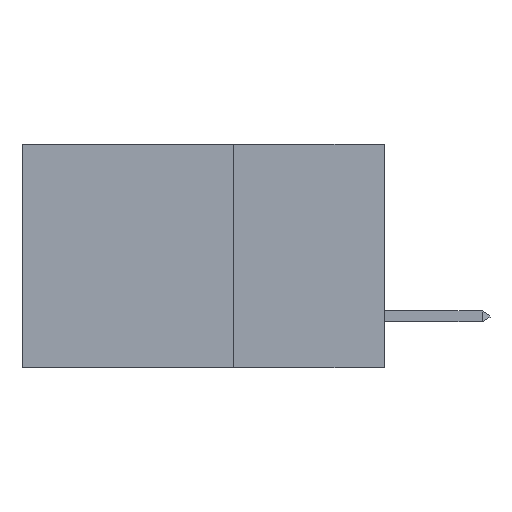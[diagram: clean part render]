
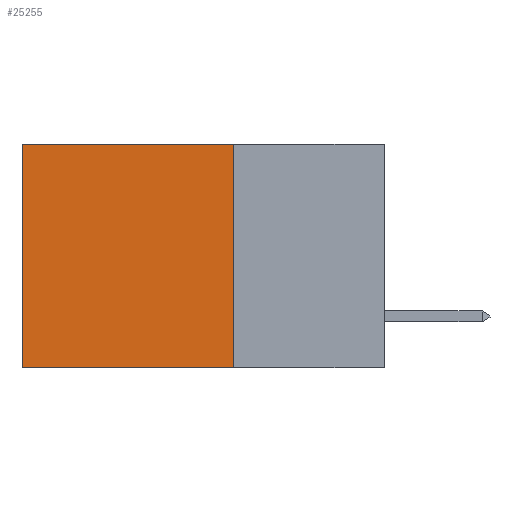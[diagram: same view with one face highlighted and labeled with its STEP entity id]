
A CAD part, left-side view. The second image highlights one B-rep face of the part: STEP entity #25255.
In plain terms, the highlighted planar face has unit normal (-1, 0, 0).
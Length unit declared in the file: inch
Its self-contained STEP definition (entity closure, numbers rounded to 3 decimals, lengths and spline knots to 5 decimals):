
#588 = VECTOR ( 'NONE', #9904, 39.37008 ) ;
#791 = VECTOR ( 'NONE', #5241, 39.37008 ) ;
#2465 = CARTESIAN_POINT ( 'NONE',  ( 0.2875, 0.25, 0. ) ) ;
#3075 = VERTEX_POINT ( 'NONE', #4162 ) ;
#3774 = EDGE_CURVE ( 'NONE', #3075, #12384, #28865, .T. ) ;
#4059 = EDGE_CURVE ( 'NONE', #33000, #33064, #5730, .T. ) ;
#4162 = CARTESIAN_POINT ( 'NONE',  ( 0.2875, 0.25, -0.37 ) ) ;
#5241 = DIRECTION ( 'NONE',  ( 0., 0., -1. ) ) ;
#5730 = LINE ( 'NONE', #24574, #19468 ) ;
#6509 = CARTESIAN_POINT ( 'NONE',  ( 0.2875, 0.6, 0. ) ) ;
#9258 = DIRECTION ( 'NONE',  ( 0., 0., -1. ) ) ;
#9904 = DIRECTION ( 'NONE',  ( 0., 1., 0. ) ) ;
#10847 = DIRECTION ( 'NONE',  ( 0., 1., 0. ) ) ;
#11724 = PLANE ( 'NONE',  #21903 ) ;
#12256 = EDGE_CURVE ( 'NONE', #33064, #12384, #34961, .T. ) ;
#12384 = VERTEX_POINT ( 'NONE', #20733 ) ;
#13897 = FACE_OUTER_BOUND ( 'NONE', #34605, .T. ) ;
#14492 = DIRECTION ( 'NONE',  ( 1., 0., 0. ) ) ;
#14538 = ORIENTED_EDGE ( 'NONE', *, *, #3774, .F. ) ;
#16314 = CARTESIAN_POINT ( 'NONE',  ( 0.2875, 0.25, 0. ) ) ;
#18143 = ORIENTED_EDGE ( 'NONE', *, *, #34585, .F. ) ;
#19468 = VECTOR ( 'NONE', #10847, 39.37008 ) ;
#20733 = CARTESIAN_POINT ( 'NONE',  ( 0.2875, 0.6, -0.37 ) ) ;
#21903 = AXIS2_PLACEMENT_3D ( 'NONE', #28057, #14492, #33472 ) ;
#22027 = CARTESIAN_POINT ( 'NONE',  ( 0.2875, 0.6, 0. ) ) ;
#22685 = LINE ( 'NONE', #2465, #791 ) ;
#24574 = CARTESIAN_POINT ( 'NONE',  ( 0.2875, 0.25, 0. ) ) ;
#25255 = ADVANCED_FACE ( 'NONE', ( #13897 ), #11724, .F. ) ;
#25980 = ORIENTED_EDGE ( 'NONE', *, *, #12256, .T. ) ;
#28032 = ORIENTED_EDGE ( 'NONE', *, *, #4059, .T. ) ;
#28057 = CARTESIAN_POINT ( 'NONE',  ( 0.2875, 0.25, 0. ) ) ;
#28865 = LINE ( 'NONE', #28999, #588 ) ;
#28999 = CARTESIAN_POINT ( 'NONE',  ( 0.2875, 0.25, -0.37 ) ) ;
#33000 = VERTEX_POINT ( 'NONE', #16314 ) ;
#33064 = VERTEX_POINT ( 'NONE', #22027 ) ;
#33472 = DIRECTION ( 'NONE',  ( 0., 0., -1. ) ) ;
#34090 = VECTOR ( 'NONE', #9258, 39.37008 ) ;
#34585 = EDGE_CURVE ( 'NONE', #33000, #3075, #22685, .T. ) ;
#34605 = EDGE_LOOP ( 'NONE', ( #25980, #14538, #18143, #28032 ) ) ;
#34961 = LINE ( 'NONE', #6509, #34090 ) ;
